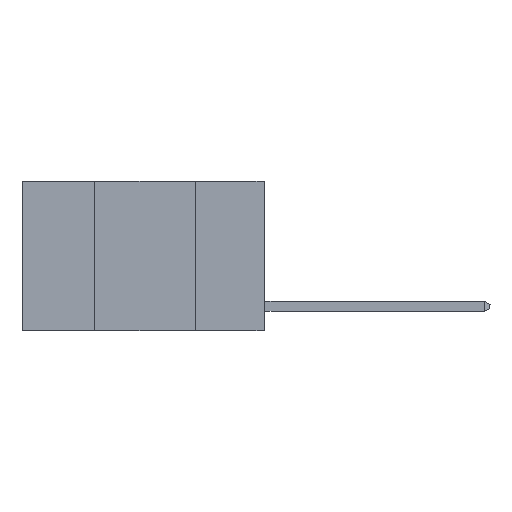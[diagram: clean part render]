
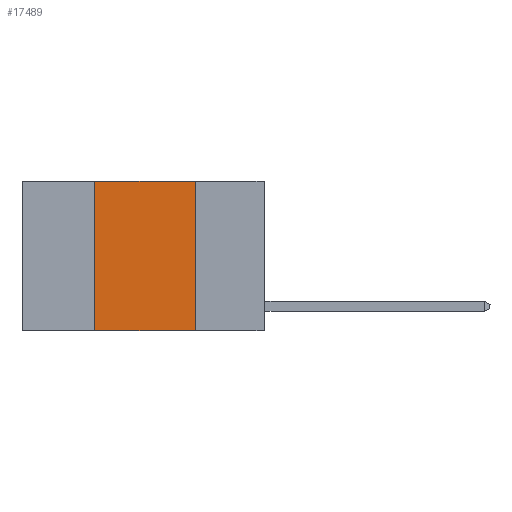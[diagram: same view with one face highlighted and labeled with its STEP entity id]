
A CAD part, left-side view. The second image highlights one B-rep face of the part: STEP entity #17489.
In plain terms, the highlighted planar face has unit normal (-1, 0, 0).
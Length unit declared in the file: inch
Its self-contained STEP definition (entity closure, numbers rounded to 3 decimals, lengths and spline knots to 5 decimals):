
#169 = VERTEX_POINT ( 'NONE', #15187 ) ;
#1636 = VECTOR ( 'NONE', #16689, 39.37008 ) ;
#2847 = CARTESIAN_POINT ( 'NONE',  ( 0., 0.42, 0. ) ) ;
#7702 = LINE ( 'NONE', #25646, #23070 ) ;
#7791 = LINE ( 'NONE', #21785, #8446 ) ;
#8446 = VECTOR ( 'NONE', #15496, 39.37008 ) ;
#9126 = EDGE_CURVE ( 'NONE', #19633, #11047, #7791, .T. ) ;
#11047 = VERTEX_POINT ( 'NONE', #11374 ) ;
#11374 = CARTESIAN_POINT ( 'NONE',  ( 0., 0.17, -0.37 ) ) ;
#11471 = CARTESIAN_POINT ( 'NONE',  ( 0., 0.6, 0. ) ) ;
#11887 = ORIENTED_EDGE ( 'NONE', *, *, #18873, .F. ) ;
#13367 = VECTOR ( 'NONE', #15255, 39.37008 ) ;
#14241 = DIRECTION ( 'NONE',  ( 0., -1., 0. ) ) ;
#14752 = EDGE_LOOP ( 'NONE', ( #23275, #24613, #11887, #15835 ) ) ;
#15187 = CARTESIAN_POINT ( 'NONE',  ( 0., 0.42, -0.37 ) ) ;
#15255 = DIRECTION ( 'NONE',  ( 0., -1., 0. ) ) ;
#15496 = DIRECTION ( 'NONE',  ( 0., 0., -1. ) ) ;
#15835 = ORIENTED_EDGE ( 'NONE', *, *, #20114, .T. ) ;
#16689 = DIRECTION ( 'NONE',  ( 0., 0., 1. ) ) ;
#16724 = AXIS2_PLACEMENT_3D ( 'NONE', #11471, #20445, #20590 ) ;
#17489 = ADVANCED_FACE ( 'NONE', ( #18627 ), #30016, .F. ) ;
#17674 = VERTEX_POINT ( 'NONE', #26223 ) ;
#18627 = FACE_OUTER_BOUND ( 'NONE', #14752, .T. ) ;
#18873 = EDGE_CURVE ( 'NONE', #169, #17674, #28253, .T. ) ;
#19633 = VERTEX_POINT ( 'NONE', #24797 ) ;
#19672 = CARTESIAN_POINT ( 'NONE',  ( 0., 0.6, 0. ) ) ;
#20114 = EDGE_CURVE ( 'NONE', #169, #11047, #7702, .T. ) ;
#20445 = DIRECTION ( 'NONE',  ( 1., 0., 0. ) ) ;
#20590 = DIRECTION ( 'NONE',  ( 0., 0., -1. ) ) ;
#21785 = CARTESIAN_POINT ( 'NONE',  ( 0., 0.17, 0. ) ) ;
#23070 = VECTOR ( 'NONE', #14241, 39.37008 ) ;
#23275 = ORIENTED_EDGE ( 'NONE', *, *, #9126, .F. ) ;
#24075 = LINE ( 'NONE', #19672, #13367 ) ;
#24613 = ORIENTED_EDGE ( 'NONE', *, *, #26392, .F. ) ;
#24797 = CARTESIAN_POINT ( 'NONE',  ( 0., 0.17, 0. ) ) ;
#25646 = CARTESIAN_POINT ( 'NONE',  ( 0., 0.6, -0.37 ) ) ;
#26223 = CARTESIAN_POINT ( 'NONE',  ( 0., 0.42, 0. ) ) ;
#26392 = EDGE_CURVE ( 'NONE', #17674, #19633, #24075, .T. ) ;
#28253 = LINE ( 'NONE', #2847, #1636 ) ;
#30016 = PLANE ( 'NONE',  #16724 ) ;
